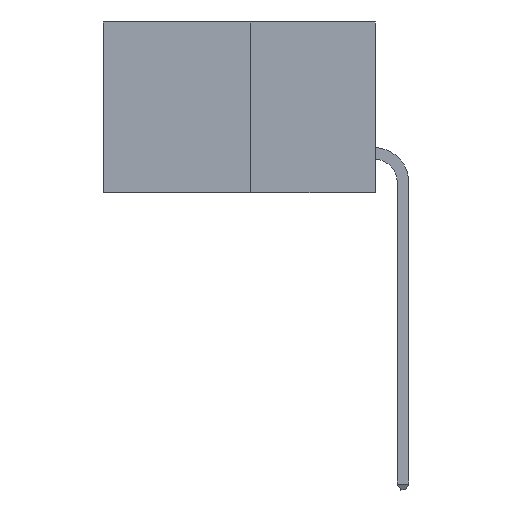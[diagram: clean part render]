
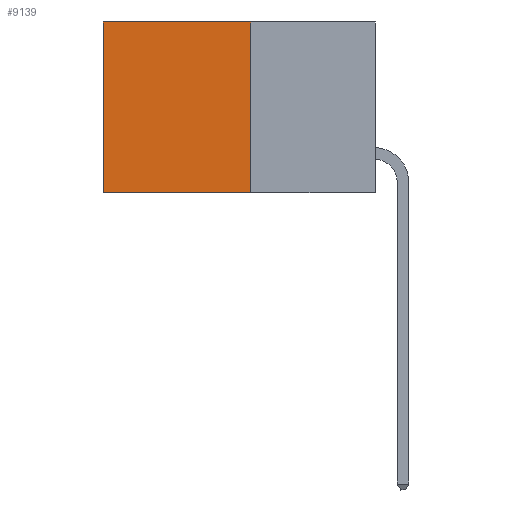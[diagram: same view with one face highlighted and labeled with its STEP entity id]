
A CAD part, left-side view. The second image highlights one B-rep face of the part: STEP entity #9139.
In plain terms, the highlighted planar face has unit normal (-1, 0, 0).
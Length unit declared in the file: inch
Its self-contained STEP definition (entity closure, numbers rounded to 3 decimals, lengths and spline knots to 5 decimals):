
#10 = LINE ( 'NONE', #8707, #14308 ) ;
#30 = VECTOR ( 'NONE', #11320, 39.37008 ) ;
#575 = EDGE_CURVE ( 'NONE', #13231, #12426, #9088, .T. ) ;
#754 = CARTESIAN_POINT ( 'NONE',  ( 0.277, 0.59, 0. ) ) ;
#932 = AXIS2_PLACEMENT_3D ( 'NONE', #5358, #13075, #6491 ) ;
#1816 = EDGE_CURVE ( 'NONE', #13231, #9473, #10, .T. ) ;
#2266 = DIRECTION ( 'NONE',  ( 0., 0., -1. ) ) ;
#3269 = VERTEX_POINT ( 'NONE', #12479 ) ;
#3820 = EDGE_CURVE ( 'NONE', #9473, #3269, #6661, .T. ) ;
#3856 = EDGE_CURVE ( 'NONE', #12426, #3269, #14643, .T. ) ;
#4027 = CARTESIAN_POINT ( 'NONE',  ( 0.277, 0.27, 0. ) ) ;
#4141 = EDGE_LOOP ( 'NONE', ( #12304, #5457, #4357, #14243 ) ) ;
#4357 = ORIENTED_EDGE ( 'NONE', *, *, #575, .F. ) ;
#5358 = CARTESIAN_POINT ( 'NONE',  ( 0.277, 0.27, -0.37 ) ) ;
#5457 = ORIENTED_EDGE ( 'NONE', *, *, #3856, .F. ) ;
#5856 = CARTESIAN_POINT ( 'NONE',  ( 0.277, 0.27, -0.37 ) ) ;
#6183 = VECTOR ( 'NONE', #2266, 39.37008 ) ;
#6491 = DIRECTION ( 'NONE',  ( 0., 0., -1. ) ) ;
#6661 = LINE ( 'NONE', #10496, #30 ) ;
#8707 = CARTESIAN_POINT ( 'NONE',  ( 0.277, 0.27, 0. ) ) ;
#8948 = FACE_OUTER_BOUND ( 'NONE', #4141, .T. ) ;
#9088 = LINE ( 'NONE', #10425, #6183 ) ;
#9139 = ADVANCED_FACE ( 'NONE', ( #8948 ), #10850, .F. ) ;
#9473 = VERTEX_POINT ( 'NONE', #754 ) ;
#10425 = CARTESIAN_POINT ( 'NONE',  ( 0.277, 0.27, -0.37 ) ) ;
#10496 = CARTESIAN_POINT ( 'NONE',  ( 0.277, 0.59, -0.37 ) ) ;
#10850 = PLANE ( 'NONE',  #932 ) ;
#11320 = DIRECTION ( 'NONE',  ( 0., 0., -1. ) ) ;
#12038 = DIRECTION ( 'NONE',  ( 0., 1., 0. ) ) ;
#12304 = ORIENTED_EDGE ( 'NONE', *, *, #3820, .T. ) ;
#12426 = VERTEX_POINT ( 'NONE', #13955 ) ;
#12479 = CARTESIAN_POINT ( 'NONE',  ( 0.277, 0.59, -0.37 ) ) ;
#13075 = DIRECTION ( 'NONE',  ( 1., 0., 0. ) ) ;
#13231 = VERTEX_POINT ( 'NONE', #4027 ) ;
#13580 = DIRECTION ( 'NONE',  ( 0., 1., 0. ) ) ;
#13955 = CARTESIAN_POINT ( 'NONE',  ( 0.277, 0.27, -0.37 ) ) ;
#14243 = ORIENTED_EDGE ( 'NONE', *, *, #1816, .T. ) ;
#14308 = VECTOR ( 'NONE', #13580, 39.37008 ) ;
#14321 = VECTOR ( 'NONE', #12038, 39.37008 ) ;
#14643 = LINE ( 'NONE', #5856, #14321 ) ;
